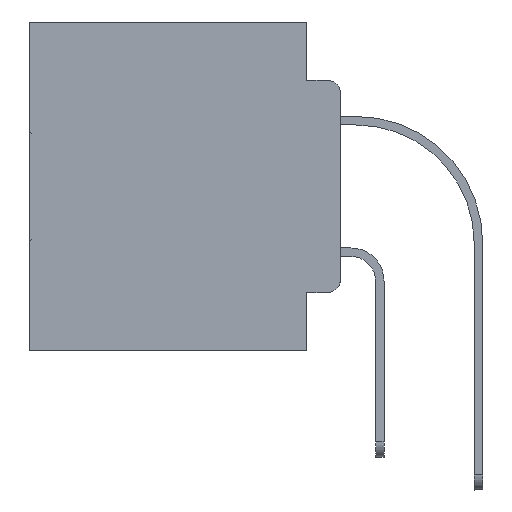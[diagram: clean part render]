
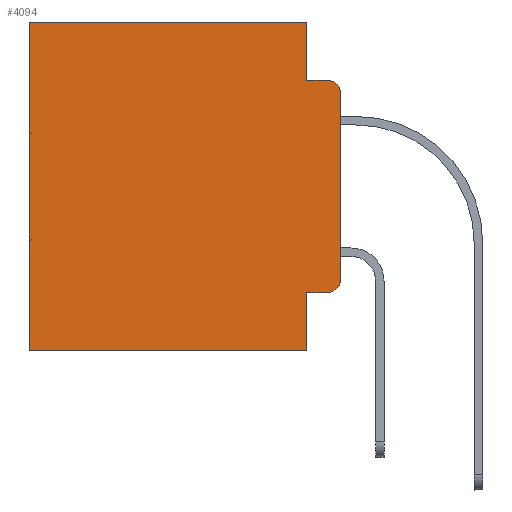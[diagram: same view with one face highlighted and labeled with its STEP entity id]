
A CAD part, left-side view. The second image highlights one B-rep face of the part: STEP entity #4094.
In plain terms, the highlighted planar face has unit normal (-1, 0, 0).
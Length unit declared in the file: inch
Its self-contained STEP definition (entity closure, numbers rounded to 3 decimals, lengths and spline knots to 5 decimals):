
#355 = EDGE_CURVE ( 'NONE', #31538, #1731, #13438, .T. ) ;
#737 = DIRECTION ( 'NONE',  ( -1., 0., 0. ) ) ;
#863 = DIRECTION ( 'NONE',  ( 0., 0., -1. ) ) ;
#897 = LINE ( 'NONE', #21206, #17470 ) ;
#1081 = DIRECTION ( 'NONE',  ( 1., 0., 0. ) ) ;
#1179 = ORIENTED_EDGE ( 'NONE', *, *, #26275, .F. ) ;
#1545 = VECTOR ( 'NONE', #8371, 39.37008 ) ;
#1731 = VERTEX_POINT ( 'NONE', #33048 ) ;
#2144 = ORIENTED_EDGE ( 'NONE', *, *, #21812, .F. ) ;
#2554 = VECTOR ( 'NONE', #863, 39.37008 ) ;
#2651 = LINE ( 'NONE', #23308, #10759 ) ;
#2799 = CARTESIAN_POINT ( 'NONE',  ( 0.298, 0.02, -0.1085 ) ) ;
#3143 = DIRECTION ( 'NONE',  ( 0., 0., -1. ) ) ;
#3369 = VERTEX_POINT ( 'NONE', #7690 ) ;
#3479 = CARTESIAN_POINT ( 'NONE',  ( 0.298, 0.051, 0. ) ) ;
#3670 = CARTESIAN_POINT ( 'NONE',  ( 0.298, 0., 0. ) ) ;
#4094 = ADVANCED_FACE ( 'NONE', ( #16715 ), #32522, .F. ) ;
#4155 = VERTEX_POINT ( 'NONE', #25831 ) ;
#4180 = AXIS2_PLACEMENT_3D ( 'NONE', #14572, #30210, #27474 ) ;
#6602 = DIRECTION ( 'NONE',  ( 0., 0., -1. ) ) ;
#6724 = CARTESIAN_POINT ( 'NONE',  ( 0.298, 0., 0. ) ) ;
#7690 = CARTESIAN_POINT ( 'NONE',  ( 0.298, 0.473, 0. ) ) ;
#8045 = CARTESIAN_POINT ( 'NONE',  ( 0.298, 0.051, 0. ) ) ;
#8069 = ORIENTED_EDGE ( 'NONE', *, *, #355, .T. ) ;
#8371 = DIRECTION ( 'NONE',  ( 0., -1., 0. ) ) ;
#8530 = VERTEX_POINT ( 'NONE', #31004 ) ;
#9377 = VERTEX_POINT ( 'NONE', #11853 ) ;
#9655 = EDGE_CURVE ( 'NONE', #10484, #12475, #16093, .T. ) ;
#10106 = EDGE_CURVE ( 'NONE', #3369, #4155, #897, .T. ) ;
#10484 = VERTEX_POINT ( 'NONE', #23912 ) ;
#10759 = VECTOR ( 'NONE', #28785, 39.37008 ) ;
#11235 = ORIENTED_EDGE ( 'NONE', *, *, #9655, .T. ) ;
#11252 = EDGE_CURVE ( 'NONE', #31699, #3369, #24938, .T. ) ;
#11853 = CARTESIAN_POINT ( 'NONE',  ( 0.298, 0.051, -0.5 ) ) ;
#11903 = EDGE_CURVE ( 'NONE', #30883, #1731, #2651, .T. ) ;
#12027 = EDGE_CURVE ( 'NONE', #31699, #30883, #27048, .T. ) ;
#12475 = VERTEX_POINT ( 'NONE', #26833 ) ;
#13438 = CIRCLE ( 'NONE', #22807, 0.02 ) ;
#13511 = EDGE_LOOP ( 'NONE', ( #19278, #8069, #19653, #22480, #19457, #23058, #2144, #1179, #11235, #21113 ) ) ;
#14572 = CARTESIAN_POINT ( 'NONE',  ( 0.298, 0.02, -0.3915 ) ) ;
#16093 = LINE ( 'NONE', #26596, #1545 ) ;
#16521 = VECTOR ( 'NONE', #22334, 39.37008 ) ;
#16531 = EDGE_CURVE ( 'NONE', #31538, #8530, #30563, .T. ) ;
#16715 = FACE_OUTER_BOUND ( 'NONE', #13511, .T. ) ;
#17470 = VECTOR ( 'NONE', #31670, 39.37008 ) ;
#19278 = ORIENTED_EDGE ( 'NONE', *, *, #16531, .F. ) ;
#19319 = VECTOR ( 'NONE', #29973, 39.37008 ) ;
#19457 = ORIENTED_EDGE ( 'NONE', *, *, #11252, .T. ) ;
#19653 = ORIENTED_EDGE ( 'NONE', *, *, #11903, .F. ) ;
#19767 = LINE ( 'NONE', #29739, #2554 ) ;
#21113 = ORIENTED_EDGE ( 'NONE', *, *, #25545, .T. ) ;
#21206 = CARTESIAN_POINT ( 'NONE',  ( 0.298, 0.473, 0. ) ) ;
#21812 = EDGE_CURVE ( 'NONE', #9377, #4155, #24484, .T. ) ;
#22197 = VECTOR ( 'NONE', #24427, 39.37008 ) ;
#22334 = DIRECTION ( 'NONE',  ( 0., 0., -1. ) ) ;
#22480 = ORIENTED_EDGE ( 'NONE', *, *, #12027, .F. ) ;
#22807 = AXIS2_PLACEMENT_3D ( 'NONE', #2799, #737, #3143 ) ;
#23058 = ORIENTED_EDGE ( 'NONE', *, *, #10106, .T. ) ;
#23308 = CARTESIAN_POINT ( 'NONE',  ( 0.298, 0.051, -0.0885 ) ) ;
#23912 = CARTESIAN_POINT ( 'NONE',  ( 0.298, 0.051, -0.4115 ) ) ;
#24427 = DIRECTION ( 'NONE',  ( 0., 1., 0. ) ) ;
#24484 = LINE ( 'NONE', #24993, #19319 ) ;
#24938 = LINE ( 'NONE', #6724, #22197 ) ;
#24993 = CARTESIAN_POINT ( 'NONE',  ( 0.298, 0., -0.5 ) ) ;
#25545 = EDGE_CURVE ( 'NONE', #12475, #8530, #32114, .T. ) ;
#25831 = CARTESIAN_POINT ( 'NONE',  ( 0.298, 0.473, -0.5 ) ) ;
#26275 = EDGE_CURVE ( 'NONE', #10484, #9377, #19767, .T. ) ;
#26596 = CARTESIAN_POINT ( 'NONE',  ( 0.298, 0.051, -0.4115 ) ) ;
#26833 = CARTESIAN_POINT ( 'NONE',  ( 0.298, 0.02, -0.4115 ) ) ;
#26870 = DIRECTION ( 'NONE',  ( 0., 0., -1. ) ) ;
#27048 = LINE ( 'NONE', #3479, #27809 ) ;
#27320 = AXIS2_PLACEMENT_3D ( 'NONE', #3670, #1081, #6602 ) ;
#27474 = DIRECTION ( 'NONE',  ( 0., 0., -1. ) ) ;
#27809 = VECTOR ( 'NONE', #26870, 39.37008 ) ;
#28785 = DIRECTION ( 'NONE',  ( 0., -1., 0. ) ) ;
#29739 = CARTESIAN_POINT ( 'NONE',  ( 0.298, 0.051, 0. ) ) ;
#29973 = DIRECTION ( 'NONE',  ( 0., 1., 0. ) ) ;
#30210 = DIRECTION ( 'NONE',  ( -1., 0., 0. ) ) ;
#30215 = CARTESIAN_POINT ( 'NONE',  ( 0.298, 0., 0. ) ) ;
#30563 = LINE ( 'NONE', #30215, #16521 ) ;
#30883 = VERTEX_POINT ( 'NONE', #31869 ) ;
#31004 = CARTESIAN_POINT ( 'NONE',  ( 0.298, 0., -0.3915 ) ) ;
#31415 = CARTESIAN_POINT ( 'NONE',  ( 0.298, 0., -0.1085 ) ) ;
#31538 = VERTEX_POINT ( 'NONE', #31415 ) ;
#31670 = DIRECTION ( 'NONE',  ( 0., 0., -1. ) ) ;
#31699 = VERTEX_POINT ( 'NONE', #8045 ) ;
#31869 = CARTESIAN_POINT ( 'NONE',  ( 0.298, 0.051, -0.0885 ) ) ;
#32114 = CIRCLE ( 'NONE', #4180, 0.02 ) ;
#32522 = PLANE ( 'NONE',  #27320 ) ;
#33048 = CARTESIAN_POINT ( 'NONE',  ( 0.298, 0.02, -0.0885 ) ) ;
